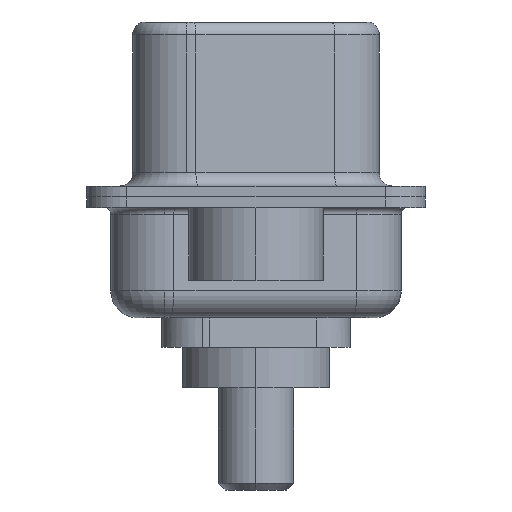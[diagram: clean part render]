
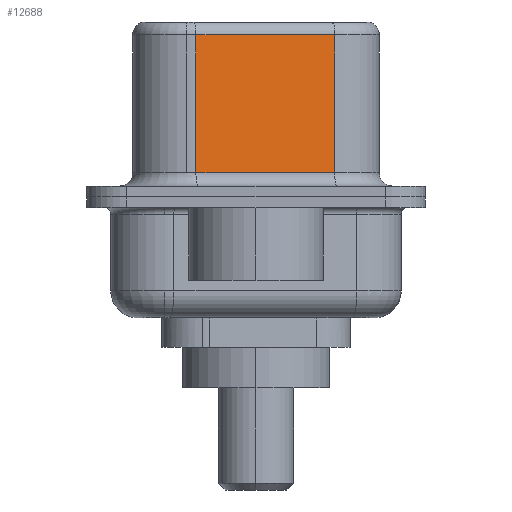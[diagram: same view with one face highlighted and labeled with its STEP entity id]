
A CAD part, left-side view. The second image highlights one B-rep face of the part: STEP entity #12688.
In plain terms, the highlighted planar face has unit normal (-0.985, -0.174, 0).
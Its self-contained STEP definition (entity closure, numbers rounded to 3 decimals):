
#21 = VERTEX_POINT ( 'NONE', #5890 ) ;
#287 = PLANE ( 'NONE',  #7410 ) ;
#1536 = ORIENTED_EDGE ( 'NONE', *, *, #2038, .F. ) ;
#1590 = LINE ( 'NONE', #12154, #7141 ) ;
#1791 = FACE_OUTER_BOUND ( 'NONE', #8338, .T. ) ;
#2038 = EDGE_CURVE ( 'NONE', #4720, #6143, #12522, .T. ) ;
#2065 = EDGE_CURVE ( 'NONE', #21, #6143, #11857, .T. ) ;
#2070 = DIRECTION ( 'NONE',  ( 0., 0., -1. ) ) ;
#2211 = EDGE_CURVE ( 'NONE', #4720, #3636, #3702, .T. ) ;
#2215 = DIRECTION ( 'NONE',  ( 0.174, -0.985, 0. ) ) ;
#2324 = CARTESIAN_POINT ( 'NONE',  ( 4.585, -2.927, 6.02 ) ) ;
#3028 = CARTESIAN_POINT ( 'NONE',  ( 4.585, -2.927, 0.9 ) ) ;
#3636 = VERTEX_POINT ( 'NONE', #12064 ) ;
#3702 = LINE ( 'NONE', #10067, #12020 ) ;
#4666 = EDGE_CURVE ( 'NONE', #3636, #21, #1590, .T. ) ;
#4720 = VERTEX_POINT ( 'NONE', #2324 ) ;
#5412 = ORIENTED_EDGE ( 'NONE', *, *, #2211, .T. ) ;
#5890 = CARTESIAN_POINT ( 'NONE',  ( 3.675, 2.233, 0.9 ) ) ;
#6012 = DIRECTION ( 'NONE',  ( 0.985, 0.174, 0. ) ) ;
#6127 = VECTOR ( 'NONE', #2215, 1000. ) ;
#6143 = VERTEX_POINT ( 'NONE', #3028 ) ;
#6449 = VECTOR ( 'NONE', #2070, 1000. ) ;
#6830 = DIRECTION ( 'NONE',  ( 0., 0., -1. ) ) ;
#7141 = VECTOR ( 'NONE', #6830, 1000. ) ;
#7410 = AXIS2_PLACEMENT_3D ( 'NONE', #12460, #6012, #13554 ) ;
#7836 = ORIENTED_EDGE ( 'NONE', *, *, #4666, .T. ) ;
#8338 = EDGE_LOOP ( 'NONE', ( #1536, #5412, #7836, #9604 ) ) ;
#9604 = ORIENTED_EDGE ( 'NONE', *, *, #2065, .T. ) ;
#10067 = CARTESIAN_POINT ( 'NONE',  ( 4.585, -2.927, 6.02 ) ) ;
#10905 = CARTESIAN_POINT ( 'NONE',  ( 4.585, -2.927, 0.9 ) ) ;
#11031 = DIRECTION ( 'NONE',  ( -0.174, 0.985, 0. ) ) ;
#11857 = LINE ( 'NONE', #10905, #6127 ) ;
#11999 = CARTESIAN_POINT ( 'NONE',  ( 4.585, -2.927, 6.52 ) ) ;
#12020 = VECTOR ( 'NONE', #11031, 1000. ) ;
#12064 = CARTESIAN_POINT ( 'NONE',  ( 3.675, 2.233, 6.02 ) ) ;
#12154 = CARTESIAN_POINT ( 'NONE',  ( 3.675, 2.233, 6.52 ) ) ;
#12460 = CARTESIAN_POINT ( 'NONE',  ( 4.585, -2.927, 6.52 ) ) ;
#12522 = LINE ( 'NONE', #11999, #6449 ) ;
#12688 = ADVANCED_FACE ( 'NONE', ( #1791 ), #287, .F. ) ;
#13554 = DIRECTION ( 'NONE',  ( -0.174, 0.985, 0. ) ) ;
